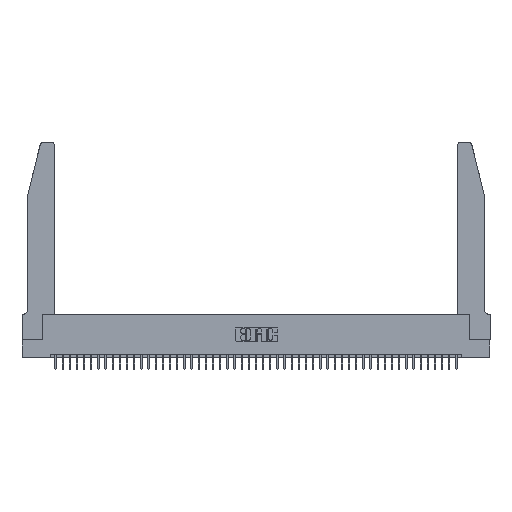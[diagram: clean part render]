
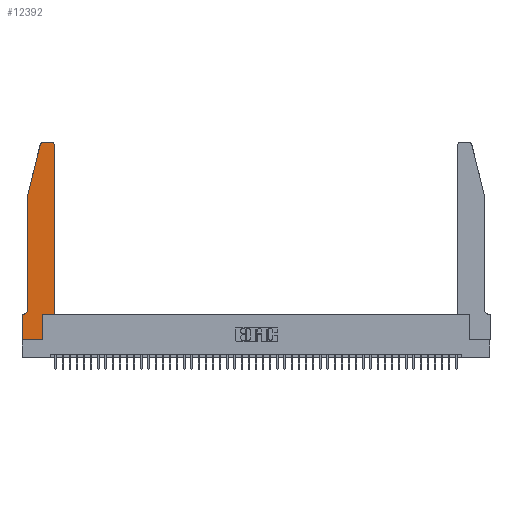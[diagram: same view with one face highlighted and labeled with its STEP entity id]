
A CAD part, top view. The second image highlights one B-rep face of the part: STEP entity #12392.
In plain terms, the highlighted planar face has unit normal (0, 0, 1).
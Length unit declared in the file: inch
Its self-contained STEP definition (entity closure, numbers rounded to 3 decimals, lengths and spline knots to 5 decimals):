
#259 = CARTESIAN_POINT ( 'NONE',  ( 0.0055, 0.35, 0.37 ) ) ;
#305 = VERTEX_POINT ( 'NONE', #30860 ) ;
#1764 = VERTEX_POINT ( 'NONE', #26220 ) ;
#2254 = EDGE_CURVE ( 'NONE', #33450, #1764, #2567, .T. ) ;
#2567 = LINE ( 'NONE', #42133, #32418 ) ;
#2796 = EDGE_CURVE ( 'NONE', #1764, #19380, #23174, .T. ) ;
#3796 = CARTESIAN_POINT ( 'NONE',  ( 0.0755, 2., 0.37 ) ) ;
#4628 = VERTEX_POINT ( 'NONE', #11921 ) ;
#4656 = CARTESIAN_POINT ( 'NONE',  ( 0.4505, 0.35, 0.37 ) ) ;
#5300 = VERTEX_POINT ( 'NONE', #3796 ) ;
#5445 = DIRECTION ( 'NONE',  ( 0., -1., 0. ) ) ;
#6098 = CARTESIAN_POINT ( 'NONE',  ( 0.284, 2.75, 0.37 ) ) ;
#6188 = DIRECTION ( 'NONE',  ( 1., 0., 0. ) ) ;
#6740 = ORIENTED_EDGE ( 'NONE', *, *, #9438, .T. ) ;
#6978 = EDGE_CURVE ( 'NONE', #43680, #14875, #25716, .T. ) ;
#7554 = AXIS2_PLACEMENT_3D ( 'NONE', #21676, #43449, #39802 ) ;
#8108 = VERTEX_POINT ( 'NONE', #6098 ) ;
#8788 = VERTEX_POINT ( 'NONE', #9415 ) ;
#8820 = CARTESIAN_POINT ( 'NONE',  ( 0., 0.35, 0.37 ) ) ;
#8833 = ORIENTED_EDGE ( 'NONE', *, *, #35312, .T. ) ;
#9415 = CARTESIAN_POINT ( 'NONE',  ( 0.4205, 2.75, 0.37 ) ) ;
#9438 = EDGE_CURVE ( 'NONE', #14875, #305, #37001, .T. ) ;
#9493 = CARTESIAN_POINT ( 'NONE',  ( 0., 0.35, 0.37 ) ) ;
#10212 = VERTEX_POINT ( 'NONE', #46187 ) ;
#11099 = VECTOR ( 'NONE', #34324, 39.37008 ) ;
#11166 = VECTOR ( 'NONE', #5445, 39.37008 ) ;
#11921 = CARTESIAN_POINT ( 'NONE',  ( 0.0755, 0.42, 0.37 ) ) ;
#12392 = ADVANCED_FACE ( 'NONE', ( #26978 ), #42069, .T. ) ;
#12462 = VECTOR ( 'NONE', #18616, 39.37008 ) ;
#12587 = DIRECTION ( 'NONE',  ( 1., 0., 0. ) ) ;
#13715 = CARTESIAN_POINT ( 'NONE',  ( 0.4505, 0.35, 0.37 ) ) ;
#14140 = EDGE_CURVE ( 'NONE', #8788, #8108, #27455, .T. ) ;
#14370 = CARTESIAN_POINT ( 'NONE',  ( 0.0755, 2., 0.37 ) ) ;
#14875 = VERTEX_POINT ( 'NONE', #9493 ) ;
#15070 = ORIENTED_EDGE ( 'NONE', *, *, #37542, .T. ) ;
#15445 = VECTOR ( 'NONE', #15911, 39.37008 ) ;
#15911 = DIRECTION ( 'NONE',  ( 0., 1., 0. ) ) ;
#15958 = CARTESIAN_POINT ( 'NONE',  ( 0.0755, 2., 0.37 ) ) ;
#16236 = ORIENTED_EDGE ( 'NONE', *, *, #22875, .T. ) ;
#16283 = DIRECTION ( 'NONE',  ( 0., 0., 1. ) ) ;
#17734 = DIRECTION ( 'NONE',  ( -0.239, -0.971, 0. ) ) ;
#18616 = DIRECTION ( 'NONE',  ( 1., 0., 0. ) ) ;
#18964 = CARTESIAN_POINT ( 'NONE',  ( 0., 0., 0.37 ) ) ;
#19380 = VERTEX_POINT ( 'NONE', #13715 ) ;
#19610 = DIRECTION ( 'NONE',  ( 0., 0., 1. ) ) ;
#20312 = ORIENTED_EDGE ( 'NONE', *, *, #2254, .T. ) ;
#20503 = DIRECTION ( 'NONE',  ( 0., 0., 1. ) ) ;
#20658 = CARTESIAN_POINT ( 'NONE',  ( 0.4205, 2.72, 0.37 ) ) ;
#20779 = DIRECTION ( 'NONE',  ( -1., 0., 0. ) ) ;
#21676 = CARTESIAN_POINT ( 'NONE',  ( 0.0055, 0.42, 0.37 ) ) ;
#22875 = EDGE_CURVE ( 'NONE', #8108, #43729, #40360, .T. ) ;
#22976 = CARTESIAN_POINT ( 'NONE',  ( 0.284, 2.72, 0.37 ) ) ;
#23174 = LINE ( 'NONE', #4656, #11099 ) ;
#23860 = DIRECTION ( 'NONE',  ( 0., 1., 0. ) ) ;
#24558 = LINE ( 'NONE', #40564, #12462 ) ;
#25716 = LINE ( 'NONE', #30832, #33150 ) ;
#26187 = ORIENTED_EDGE ( 'NONE', *, *, #32921, .T. ) ;
#26220 = CARTESIAN_POINT ( 'NONE',  ( 0.2865, 0.35, 0.37 ) ) ;
#26958 = EDGE_LOOP ( 'NONE', ( #44320, #16236, #45190, #8833, #32423, #32679, #6740, #46815, #20312, #30749, #15070, #26187 ) ) ;
#26978 = FACE_OUTER_BOUND ( 'NONE', #26958, .T. ) ;
#27169 = DIRECTION ( 'NONE',  ( -1., 0., 0. ) ) ;
#27455 = LINE ( 'NONE', #46100, #46965 ) ;
#27496 = VECTOR ( 'NONE', #17734, 39.37008 ) ;
#27946 = CIRCLE ( 'NONE', #7554, 0.07 ) ;
#29464 = AXIS2_PLACEMENT_3D ( 'NONE', #22976, #19610, #34497 ) ;
#30749 = ORIENTED_EDGE ( 'NONE', *, *, #2796, .T. ) ;
#30832 = CARTESIAN_POINT ( 'NONE',  ( 0.0755, 0.35, 0.37 ) ) ;
#30860 = CARTESIAN_POINT ( 'NONE',  ( 0., 0., 0.37 ) ) ;
#32418 = VECTOR ( 'NONE', #23860, 39.37008 ) ;
#32423 = ORIENTED_EDGE ( 'NONE', *, *, #34309, .T. ) ;
#32679 = ORIENTED_EDGE ( 'NONE', *, *, #6978, .T. ) ;
#32921 = EDGE_CURVE ( 'NONE', #10212, #8788, #34965, .T. ) ;
#33150 = VECTOR ( 'NONE', #27169, 39.37008 ) ;
#33186 = CARTESIAN_POINT ( 'NONE',  ( 0.25487, 2.72718, 0.37 ) ) ;
#33450 = VERTEX_POINT ( 'NONE', #41281 ) ;
#33893 = DIRECTION ( 'NONE',  ( 0., -1., 0. ) ) ;
#34309 = EDGE_CURVE ( 'NONE', #4628, #43680, #27946, .T. ) ;
#34324 = DIRECTION ( 'NONE',  ( 1., 0., 0. ) ) ;
#34497 = DIRECTION ( 'NONE',  ( 1., 0., 0. ) ) ;
#34965 = CIRCLE ( 'NONE', #37283, 0.03 ) ;
#35312 = EDGE_CURVE ( 'NONE', #5300, #4628, #47130, .T. ) ;
#37001 = LINE ( 'NONE', #18964, #11166 ) ;
#37200 = EDGE_CURVE ( 'NONE', #43729, #5300, #38993, .T. ) ;
#37283 = AXIS2_PLACEMENT_3D ( 'NONE', #20658, #20503, #6188 ) ;
#37352 = VECTOR ( 'NONE', #33893, 39.37008 ) ;
#37377 = CARTESIAN_POINT ( 'NONE',  ( 0.4505, 0.35, 0.37 ) ) ;
#37542 = EDGE_CURVE ( 'NONE', #19380, #10212, #38950, .T. ) ;
#38394 = EDGE_CURVE ( 'NONE', #305, #33450, #24558, .T. ) ;
#38950 = LINE ( 'NONE', #37377, #15445 ) ;
#38993 = LINE ( 'NONE', #14370, #27496 ) ;
#39802 = DIRECTION ( 'NONE',  ( -1., 0., 0. ) ) ;
#40360 = CIRCLE ( 'NONE', #29464, 0.03 ) ;
#40564 = CARTESIAN_POINT ( 'NONE',  ( 0., 0., 0.37 ) ) ;
#41281 = CARTESIAN_POINT ( 'NONE',  ( 0.2865, 0., 0.37 ) ) ;
#42069 = PLANE ( 'NONE',  #47032 ) ;
#42133 = CARTESIAN_POINT ( 'NONE',  ( 0.2865, 0.35, 0.37 ) ) ;
#43449 = DIRECTION ( 'NONE',  ( 0., 0., -1. ) ) ;
#43680 = VERTEX_POINT ( 'NONE', #259 ) ;
#43729 = VERTEX_POINT ( 'NONE', #33186 ) ;
#44320 = ORIENTED_EDGE ( 'NONE', *, *, #14140, .T. ) ;
#45190 = ORIENTED_EDGE ( 'NONE', *, *, #37200, .T. ) ;
#46100 = CARTESIAN_POINT ( 'NONE',  ( 0.2605, 2.75, 0.37 ) ) ;
#46187 = CARTESIAN_POINT ( 'NONE',  ( 0.4505, 2.72, 0.37 ) ) ;
#46815 = ORIENTED_EDGE ( 'NONE', *, *, #38394, .T. ) ;
#46965 = VECTOR ( 'NONE', #20779, 39.37008 ) ;
#47032 = AXIS2_PLACEMENT_3D ( 'NONE', #8820, #16283, #12587 ) ;
#47130 = LINE ( 'NONE', #15958, #37352 ) ;
